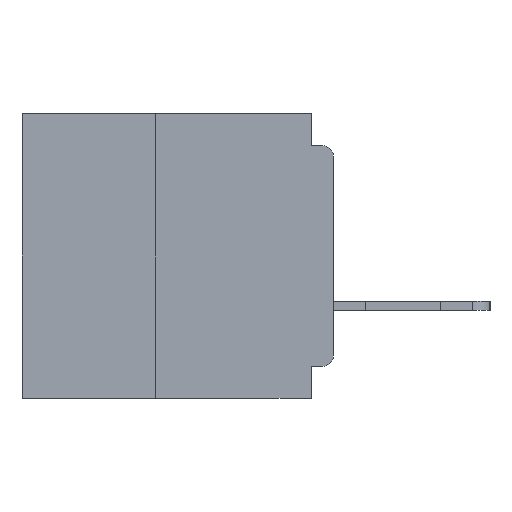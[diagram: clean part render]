
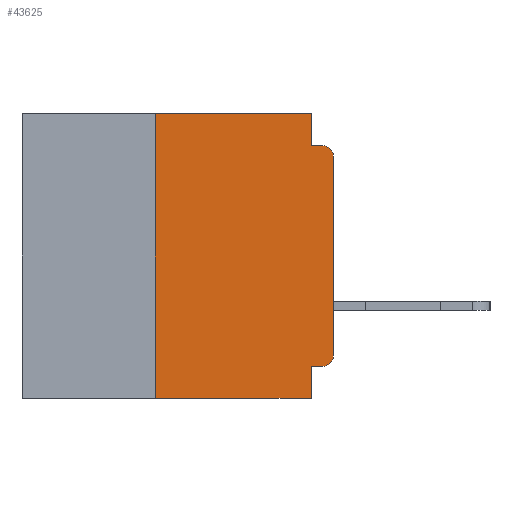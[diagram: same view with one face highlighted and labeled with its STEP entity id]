
A CAD part, left-side view. The second image highlights one B-rep face of the part: STEP entity #43625.
In plain terms, the highlighted planar face has unit normal (-1, 0, 0).
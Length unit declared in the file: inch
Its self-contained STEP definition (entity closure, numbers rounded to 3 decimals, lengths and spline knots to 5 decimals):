
#358 = EDGE_CURVE ( 'NONE', #48322, #34629, #18351, .T. ) ;
#1191 = LINE ( 'NONE', #38154, #9432 ) ;
#1301 = CARTESIAN_POINT ( 'NONE',  ( 0., 0.031, -0.4 ) ) ;
#2446 = EDGE_CURVE ( 'NONE', #17608, #48322, #44845, .T. ) ;
#2479 = LINE ( 'NONE', #41230, #13271 ) ;
#2905 = DIRECTION ( 'NONE',  ( 0., 0., -1. ) ) ;
#2924 = VECTOR ( 'NONE', #5450, 39.37008 ) ;
#2961 = VERTEX_POINT ( 'NONE', #25284 ) ;
#3390 = CARTESIAN_POINT ( 'NONE',  ( 0., 0.031, -0.355 ) ) ;
#4662 = EDGE_CURVE ( 'NONE', #20874, #49661, #40756, .T. ) ;
#5450 = DIRECTION ( 'NONE',  ( 0., 1., 0. ) ) ;
#5781 = EDGE_CURVE ( 'NONE', #33287, #34629, #37453, .T. ) ;
#9432 = VECTOR ( 'NONE', #30053, 39.37008 ) ;
#10647 = VERTEX_POINT ( 'NONE', #40831 ) ;
#10902 = CARTESIAN_POINT ( 'NONE',  ( 0., 0.015, -0.355 ) ) ;
#11573 = CIRCLE ( 'NONE', #25350, 0.015 ) ;
#12114 = ORIENTED_EDGE ( 'NONE', *, *, #20450, .T. ) ;
#12183 = LINE ( 'NONE', #52188, #20419 ) ;
#13271 = VECTOR ( 'NONE', #49420, 39.37008 ) ;
#15838 = VECTOR ( 'NONE', #27928, 39.37008 ) ;
#16621 = EDGE_CURVE ( 'NONE', #33287, #20874, #33620, .T. ) ;
#17608 = VERTEX_POINT ( 'NONE', #10902 ) ;
#18277 = ORIENTED_EDGE ( 'NONE', *, *, #2446, .F. ) ;
#18351 = LINE ( 'NONE', #23213, #52043 ) ;
#20419 = VECTOR ( 'NONE', #23971, 39.37008 ) ;
#20450 = EDGE_CURVE ( 'NONE', #31175, #2961, #12183, .T. ) ;
#20874 = VERTEX_POINT ( 'NONE', #34725 ) ;
#21624 = CARTESIAN_POINT ( 'NONE',  ( 0., 0.437, 0. ) ) ;
#21935 = CIRCLE ( 'NONE', #37377, 0.015 ) ;
#22095 = EDGE_CURVE ( 'NONE', #49661, #10647, #2479, .T. ) ;
#22266 = ORIENTED_EDGE ( 'NONE', *, *, #16621, .F. ) ;
#22632 = FACE_OUTER_BOUND ( 'NONE', #33645, .T. ) ;
#23104 = DIRECTION ( 'NONE',  ( 0., 0., -1. ) ) ;
#23213 = CARTESIAN_POINT ( 'NONE',  ( 0., 0.031, -0.4 ) ) ;
#23971 = DIRECTION ( 'NONE',  ( 0., 0., 1. ) ) ;
#24018 = DIRECTION ( 'NONE',  ( -1., 0., 0. ) ) ;
#24107 = DIRECTION ( 'NONE',  ( 0., 0., 1. ) ) ;
#25217 = EDGE_CURVE ( 'NONE', #17608, #31175, #11573, .T. ) ;
#25284 = CARTESIAN_POINT ( 'NONE',  ( 0., 0., -0.06 ) ) ;
#25350 = AXIS2_PLACEMENT_3D ( 'NONE', #48348, #24018, #52398 ) ;
#25730 = DIRECTION ( 'NONE',  ( 0., 0., -1. ) ) ;
#26141 = ORIENTED_EDGE ( 'NONE', *, *, #22095, .F. ) ;
#27263 = DIRECTION ( 'NONE',  ( -1., 0., 0. ) ) ;
#27928 = DIRECTION ( 'NONE',  ( 0., -1., 0. ) ) ;
#28740 = CARTESIAN_POINT ( 'NONE',  ( 0., 0., -0.34 ) ) ;
#28928 = DIRECTION ( 'NONE',  ( 0., -1., 0. ) ) ;
#30053 = DIRECTION ( 'NONE',  ( 0., -1., 0. ) ) ;
#31175 = VERTEX_POINT ( 'NONE', #28740 ) ;
#31600 = ORIENTED_EDGE ( 'NONE', *, *, #25217, .T. ) ;
#31778 = ORIENTED_EDGE ( 'NONE', *, *, #5781, .T. ) ;
#32313 = VECTOR ( 'NONE', #24107, 39.37008 ) ;
#33134 = ORIENTED_EDGE ( 'NONE', *, *, #358, .F. ) ;
#33252 = CARTESIAN_POINT ( 'NONE',  ( 0., 0.031, 0. ) ) ;
#33287 = VERTEX_POINT ( 'NONE', #48994 ) ;
#33620 = LINE ( 'NONE', #35971, #32313 ) ;
#33645 = EDGE_LOOP ( 'NONE', ( #12114, #37120, #40936, #26141, #47296, #22266, #31778, #33134, #18277, #31600 ) ) ;
#34629 = VERTEX_POINT ( 'NONE', #1301 ) ;
#34725 = CARTESIAN_POINT ( 'NONE',  ( 0., 0.25, 0. ) ) ;
#35971 = CARTESIAN_POINT ( 'NONE',  ( 0., 0.25, -0.4 ) ) ;
#36032 = CARTESIAN_POINT ( 'NONE',  ( 0., 0.437, -0.4 ) ) ;
#36648 = AXIS2_PLACEMENT_3D ( 'NONE', #21624, #50034, #25730 ) ;
#37120 = ORIENTED_EDGE ( 'NONE', *, *, #44261, .T. ) ;
#37377 = AXIS2_PLACEMENT_3D ( 'NONE', #51545, #27263, #2905 ) ;
#37453 = LINE ( 'NONE', #36032, #15838 ) ;
#37793 = EDGE_CURVE ( 'NONE', #10647, #47552, #1191, .T. ) ;
#37919 = CARTESIAN_POINT ( 'NONE',  ( 0., 0., -0.355 ) ) ;
#38078 = CARTESIAN_POINT ( 'NONE',  ( 0., 0.015, -0.045 ) ) ;
#38154 = CARTESIAN_POINT ( 'NONE',  ( 0., 0., -0.045 ) ) ;
#39486 = VECTOR ( 'NONE', #28928, 39.37008 ) ;
#40756 = LINE ( 'NONE', #49165, #39486 ) ;
#40831 = CARTESIAN_POINT ( 'NONE',  ( 0., 0.031, -0.045 ) ) ;
#40936 = ORIENTED_EDGE ( 'NONE', *, *, #37793, .F. ) ;
#41230 = CARTESIAN_POINT ( 'NONE',  ( 0., 0.031, 0. ) ) ;
#43625 = ADVANCED_FACE ( 'NONE', ( #22632 ), #45956, .F. ) ;
#44261 = EDGE_CURVE ( 'NONE', #2961, #47552, #21935, .T. ) ;
#44845 = LINE ( 'NONE', #37919, #2924 ) ;
#45956 = PLANE ( 'NONE',  #36648 ) ;
#47296 = ORIENTED_EDGE ( 'NONE', *, *, #4662, .F. ) ;
#47552 = VERTEX_POINT ( 'NONE', #38078 ) ;
#48322 = VERTEX_POINT ( 'NONE', #3390 ) ;
#48348 = CARTESIAN_POINT ( 'NONE',  ( 0., 0.015, -0.34 ) ) ;
#48994 = CARTESIAN_POINT ( 'NONE',  ( 0., 0.25, -0.4 ) ) ;
#49165 = CARTESIAN_POINT ( 'NONE',  ( 0., 0.437, 0. ) ) ;
#49420 = DIRECTION ( 'NONE',  ( 0., 0., -1. ) ) ;
#49661 = VERTEX_POINT ( 'NONE', #33252 ) ;
#50034 = DIRECTION ( 'NONE',  ( 1., 0., 0. ) ) ;
#51545 = CARTESIAN_POINT ( 'NONE',  ( 0., 0.015, -0.06 ) ) ;
#52043 = VECTOR ( 'NONE', #23104, 39.37008 ) ;
#52188 = CARTESIAN_POINT ( 'NONE',  ( 0., 0., 0. ) ) ;
#52398 = DIRECTION ( 'NONE',  ( 0., 0., -1. ) ) ;
